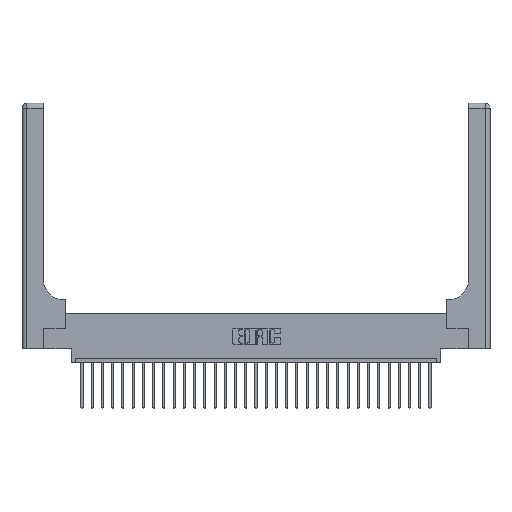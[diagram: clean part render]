
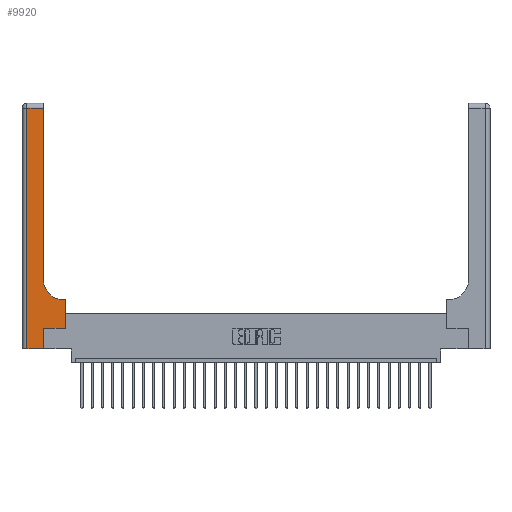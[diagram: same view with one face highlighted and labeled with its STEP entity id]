
A CAD part, top view. The second image highlights one B-rep face of the part: STEP entity #9920.
In plain terms, the highlighted planar face has unit normal (0, 0, 1).
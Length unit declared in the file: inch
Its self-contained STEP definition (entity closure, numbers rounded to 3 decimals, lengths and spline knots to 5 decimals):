
#620 = ORIENTED_EDGE ( 'NONE', *, *, #6923, .T. ) ;
#1077 = LINE ( 'NONE', #26992, #26786 ) ;
#1151 = CARTESIAN_POINT ( 'NONE',  ( 0.26, 2.94, 0.37 ) ) ;
#2194 = CARTESIAN_POINT ( 'NONE',  ( 0.06, 2.94, 0.37 ) ) ;
#2231 = CARTESIAN_POINT ( 'NONE',  ( 0.26, 0.85, 0.37 ) ) ;
#2594 = DIRECTION ( 'NONE',  ( 1., 0., 0. ) ) ;
#2650 = VECTOR ( 'NONE', #20178, 39.37008 ) ;
#3603 = DIRECTION ( 'NONE',  ( 0., 1., 0. ) ) ;
#3671 = CIRCLE ( 'NONE', #24800, 0.25 ) ;
#3785 = EDGE_CURVE ( 'NONE', #25072, #24274, #10971, .T. ) ;
#3887 = CARTESIAN_POINT ( 'NONE',  ( 0.26, 3., 0.37 ) ) ;
#4066 = DIRECTION ( 'NONE',  ( 0., 1., 0. ) ) ;
#4440 = VERTEX_POINT ( 'NONE', #22419 ) ;
#5270 = FACE_OUTER_BOUND ( 'NONE', #21614, .T. ) ;
#6058 = DIRECTION ( 'NONE',  ( 0., -1., 0. ) ) ;
#6643 = VECTOR ( 'NONE', #15303, 39.37008 ) ;
#6752 = ORIENTED_EDGE ( 'NONE', *, *, #3785, .T. ) ;
#6923 = EDGE_CURVE ( 'NONE', #4440, #12625, #3671, .T. ) ;
#7140 = AXIS2_PLACEMENT_3D ( 'NONE', #27018, #24857, #14052 ) ;
#8246 = EDGE_CURVE ( 'NONE', #12625, #25072, #27753, .T. ) ;
#8596 = CARTESIAN_POINT ( 'NONE',  ( 0.528, 0.6, 0.37 ) ) ;
#8708 = VERTEX_POINT ( 'NONE', #14922 ) ;
#8813 = CARTESIAN_POINT ( 'NONE',  ( 0.265, 0., 0.37 ) ) ;
#8954 = LINE ( 'NONE', #16282, #18337 ) ;
#9609 = PLANE ( 'NONE',  #7140 ) ;
#9920 = ADVANCED_FACE ( 'NONE', ( #5270 ), #9609, .F. ) ;
#10519 = LINE ( 'NONE', #17138, #19814 ) ;
#10771 = VERTEX_POINT ( 'NONE', #17117 ) ;
#10832 = LINE ( 'NONE', #11387, #2650 ) ;
#10882 = VERTEX_POINT ( 'NONE', #28039 ) ;
#10971 = LINE ( 'NONE', #23924, #6643 ) ;
#11345 = CARTESIAN_POINT ( 'NONE',  ( 0., 0., 0.37 ) ) ;
#11387 = CARTESIAN_POINT ( 'NONE',  ( 0.528, 0.25, 0.37 ) ) ;
#11433 = DIRECTION ( 'NONE',  ( -1., 0., 0. ) ) ;
#11807 = CARTESIAN_POINT ( 'NONE',  ( 0.51, 0.85, 0.37 ) ) ;
#11942 = VECTOR ( 'NONE', #3603, 39.37008 ) ;
#12006 = ORIENTED_EDGE ( 'NONE', *, *, #12936, .T. ) ;
#12086 = ORIENTED_EDGE ( 'NONE', *, *, #17296, .T. ) ;
#12625 = VERTEX_POINT ( 'NONE', #2231 ) ;
#12936 = EDGE_CURVE ( 'NONE', #18024, #14515, #10832, .T. ) ;
#13689 = EDGE_CURVE ( 'NONE', #10771, #10882, #26229, .T. ) ;
#13705 = EDGE_CURVE ( 'NONE', #10882, #18024, #8954, .T. ) ;
#14052 = DIRECTION ( 'NONE',  ( -1., 0., 0. ) ) ;
#14193 = VECTOR ( 'NONE', #4066, 39.37008 ) ;
#14515 = VERTEX_POINT ( 'NONE', #8596 ) ;
#14922 = CARTESIAN_POINT ( 'NONE',  ( 0.06, 0., 0.37 ) ) ;
#15303 = DIRECTION ( 'NONE',  ( -1., 0., 0. ) ) ;
#15365 = CARTESIAN_POINT ( 'NONE',  ( 0.528, 0.25, 0.37 ) ) ;
#16282 = CARTESIAN_POINT ( 'NONE',  ( 0.265, 0.25, 0.37 ) ) ;
#17117 = CARTESIAN_POINT ( 'NONE',  ( 0.265, 0., 0.37 ) ) ;
#17138 = CARTESIAN_POINT ( 'NONE',  ( 0.06, 3., 0.37 ) ) ;
#17296 = EDGE_CURVE ( 'NONE', #24274, #8708, #10519, .T. ) ;
#17594 = EDGE_CURVE ( 'NONE', #8708, #10771, #24031, .T. ) ;
#18024 = VERTEX_POINT ( 'NONE', #15365 ) ;
#18337 = VECTOR ( 'NONE', #2594, 39.37008 ) ;
#18724 = ORIENTED_EDGE ( 'NONE', *, *, #17594, .T. ) ;
#18892 = VECTOR ( 'NONE', #27045, 39.37008 ) ;
#19814 = VECTOR ( 'NONE', #6058, 39.37008 ) ;
#20178 = DIRECTION ( 'NONE',  ( 0., 1., 0. ) ) ;
#21614 = EDGE_LOOP ( 'NONE', ( #27806, #6752, #12086, #18724, #25203, #26228, #12006, #23527, #620 ) ) ;
#22419 = CARTESIAN_POINT ( 'NONE',  ( 0.51, 0.6, 0.37 ) ) ;
#23527 = ORIENTED_EDGE ( 'NONE', *, *, #27599, .T. ) ;
#23924 = CARTESIAN_POINT ( 'NONE',  ( 0., 2.94, 0.37 ) ) ;
#24031 = LINE ( 'NONE', #11345, #18892 ) ;
#24274 = VERTEX_POINT ( 'NONE', #2194 ) ;
#24800 = AXIS2_PLACEMENT_3D ( 'NONE', #11807, #25066, #25503 ) ;
#24857 = DIRECTION ( 'NONE',  ( 0., 0., -1. ) ) ;
#25066 = DIRECTION ( 'NONE',  ( 0., 0., -1. ) ) ;
#25072 = VERTEX_POINT ( 'NONE', #1151 ) ;
#25203 = ORIENTED_EDGE ( 'NONE', *, *, #13689, .T. ) ;
#25503 = DIRECTION ( 'NONE',  ( 1., 0., 0. ) ) ;
#26228 = ORIENTED_EDGE ( 'NONE', *, *, #13705, .T. ) ;
#26229 = LINE ( 'NONE', #8813, #14193 ) ;
#26786 = VECTOR ( 'NONE', #11433, 39.37008 ) ;
#26992 = CARTESIAN_POINT ( 'NONE',  ( 0.26, 0.6, 0.37 ) ) ;
#27018 = CARTESIAN_POINT ( 'NONE',  ( 0., 3., 0.37 ) ) ;
#27045 = DIRECTION ( 'NONE',  ( 1., 0., 0. ) ) ;
#27599 = EDGE_CURVE ( 'NONE', #14515, #4440, #1077, .T. ) ;
#27753 = LINE ( 'NONE', #3887, #11942 ) ;
#27806 = ORIENTED_EDGE ( 'NONE', *, *, #8246, .T. ) ;
#28039 = CARTESIAN_POINT ( 'NONE',  ( 0.265, 0.25, 0.37 ) ) ;
